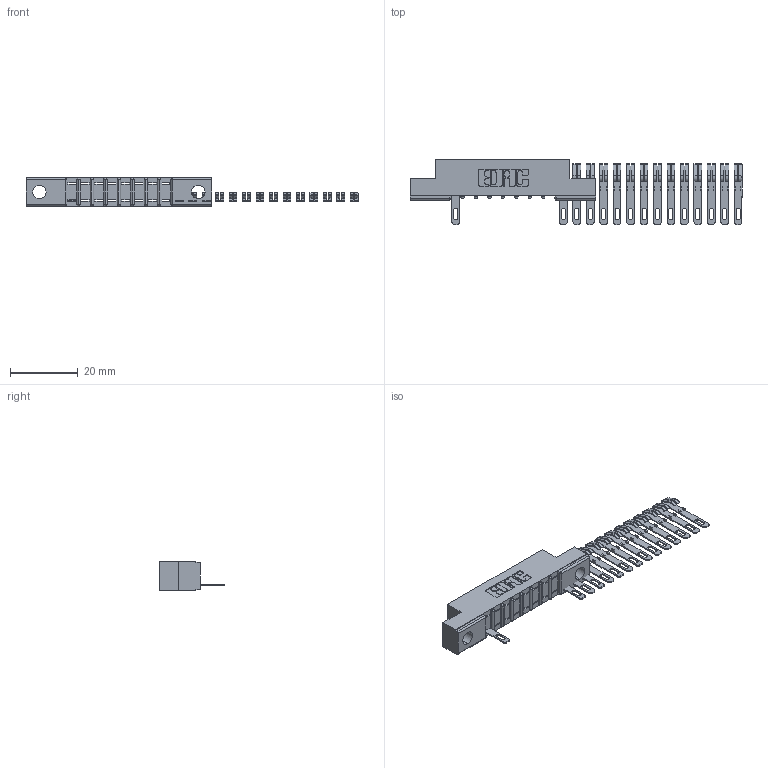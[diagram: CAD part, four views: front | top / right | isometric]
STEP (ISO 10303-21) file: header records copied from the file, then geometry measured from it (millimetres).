
FILE_DESCRIPTION (( 'STEP AP203' ), '1' );
FILE_NAME ('357-022-505-104.STEP', '2018-08-08T21:45:19', ( '' ), ( '' ), 'SwSTEP 2.0', 'SolidWorks 2016', '' );
FILE_SCHEMA (( 'CONFIG_CONTROL_DESIGN' ));
Length unit declared in the file: inch
Products named in the file (3): 307 Part_.156 Dia Mounting Holes; 307-290-001_505; 357-022-505-104
Assembly tree (16 placements, depth 2):
  357-022-505-104
    307 Part_.156 Dia Mounting Holes
    307-290-001_505  x15
Bounding box: 97.83 x 19.18 x 8.71 mm (x, y, z)
Volume: 3505.1 mm3; surface area: 5515.6 mm2
Topology: 16 solids, 16 shells, 841 faces, 2341 edges, 1514 vertices
Faces by surface type: plane 540, cylinder 283, sphere 18
Entity records: 11666 total; most frequent: CARTESIAN_POINT 1925, ORIENTED_EDGE 1902, DIRECTION 1893, EDGE_CURVE 951, LINE 721, VECTOR 721, VERTEX_POINT 618, AXIS2_PLACEMENT_3D 586
